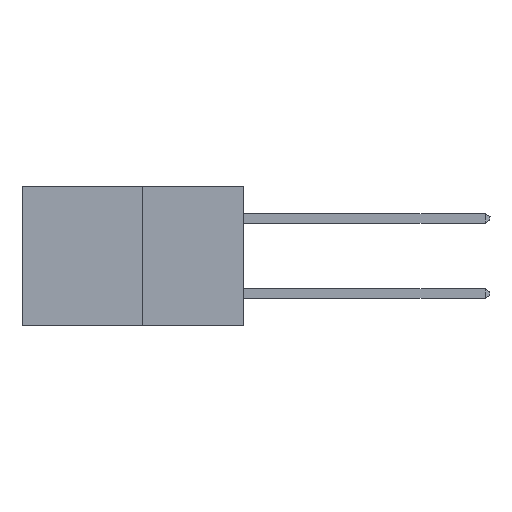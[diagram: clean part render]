
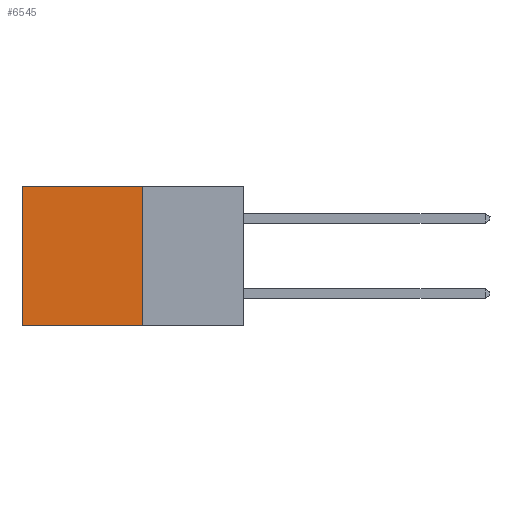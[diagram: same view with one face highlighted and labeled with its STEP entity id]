
A CAD part, left-side view. The second image highlights one B-rep face of the part: STEP entity #6545.
In plain terms, the highlighted planar face has unit normal (-1, 0, 0).
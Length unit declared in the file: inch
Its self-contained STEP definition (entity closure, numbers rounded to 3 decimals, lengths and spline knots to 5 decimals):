
#106 = VECTOR ( 'NONE', #22233, 39.37008 ) ;
#690 = EDGE_CURVE ( 'NONE', #25286, #4479, #8336, .T. ) ;
#3649 = AXIS2_PLACEMENT_3D ( 'NONE', #27450, #26576, #26572 ) ;
#4479 = VERTEX_POINT ( 'NONE', #27752 ) ;
#5740 = DIRECTION ( 'NONE',  ( 0., 1., 0. ) ) ;
#6060 = LINE ( 'NONE', #24399, #106 ) ;
#6158 = DIRECTION ( 'NONE',  ( 0., 0., -1. ) ) ;
#6218 = VERTEX_POINT ( 'NONE', #15461 ) ;
#6545 = ADVANCED_FACE ( 'NONE', ( #23863 ), #26674, .F. ) ;
#6807 = CARTESIAN_POINT ( 'NONE',  ( 0.277, 0.59, -0.37 ) ) ;
#7190 = CARTESIAN_POINT ( 'NONE',  ( 0.277, 0.27, -0.37 ) ) ;
#7329 = CARTESIAN_POINT ( 'NONE',  ( 0.277, 0.27, -0.37 ) ) ;
#8336 = LINE ( 'NONE', #6807, #19460 ) ;
#8408 = ORIENTED_EDGE ( 'NONE', *, *, #9717, .F. ) ;
#9019 = LINE ( 'NONE', #7329, #11174 ) ;
#9717 = EDGE_CURVE ( 'NONE', #10566, #4479, #6060, .T. ) ;
#9819 = CARTESIAN_POINT ( 'NONE',  ( 0.277, 0.59, 0. ) ) ;
#10102 = CARTESIAN_POINT ( 'NONE',  ( 0.277, 0.27, 0. ) ) ;
#10566 = VERTEX_POINT ( 'NONE', #7190 ) ;
#11147 = VECTOR ( 'NONE', #5740, 39.37008 ) ;
#11174 = VECTOR ( 'NONE', #22790, 39.37008 ) ;
#12868 = EDGE_CURVE ( 'NONE', #6218, #10566, #9019, .T. ) ;
#13698 = ORIENTED_EDGE ( 'NONE', *, *, #690, .T. ) ;
#15461 = CARTESIAN_POINT ( 'NONE',  ( 0.277, 0.27, 0. ) ) ;
#19460 = VECTOR ( 'NONE', #6158, 39.37008 ) ;
#22154 = EDGE_LOOP ( 'NONE', ( #13698, #8408, #26663, #25632 ) ) ;
#22233 = DIRECTION ( 'NONE',  ( 0., 1., 0. ) ) ;
#22790 = DIRECTION ( 'NONE',  ( 0., 0., -1. ) ) ;
#23230 = EDGE_CURVE ( 'NONE', #6218, #25286, #27913, .T. ) ;
#23863 = FACE_OUTER_BOUND ( 'NONE', #22154, .T. ) ;
#24399 = CARTESIAN_POINT ( 'NONE',  ( 0.277, 0.27, -0.37 ) ) ;
#25286 = VERTEX_POINT ( 'NONE', #9819 ) ;
#25632 = ORIENTED_EDGE ( 'NONE', *, *, #23230, .T. ) ;
#26572 = DIRECTION ( 'NONE',  ( 0., 0., -1. ) ) ;
#26576 = DIRECTION ( 'NONE',  ( 1., 0., 0. ) ) ;
#26663 = ORIENTED_EDGE ( 'NONE', *, *, #12868, .F. ) ;
#26674 = PLANE ( 'NONE',  #3649 ) ;
#27450 = CARTESIAN_POINT ( 'NONE',  ( 0.277, 0.27, -0.37 ) ) ;
#27752 = CARTESIAN_POINT ( 'NONE',  ( 0.277, 0.59, -0.37 ) ) ;
#27913 = LINE ( 'NONE', #10102, #11147 ) ;
